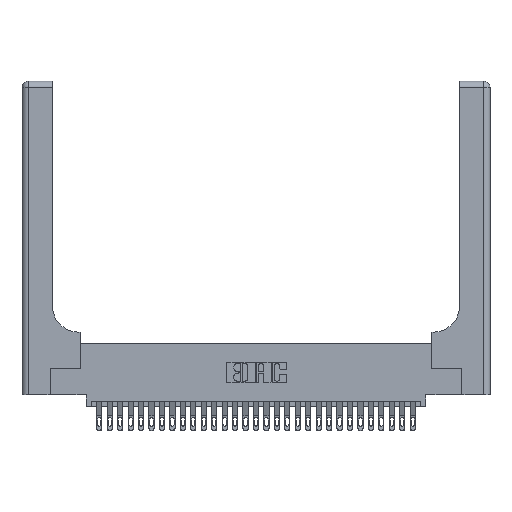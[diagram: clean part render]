
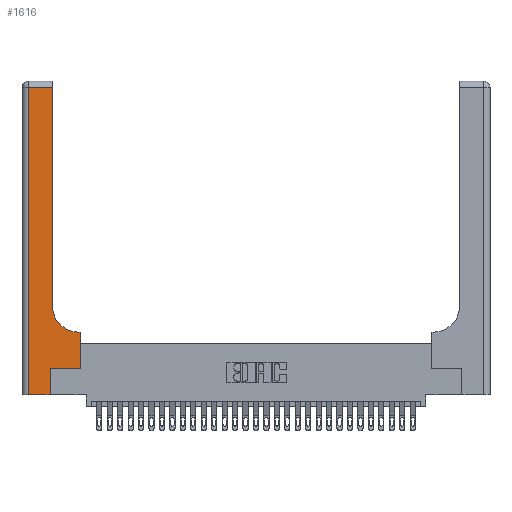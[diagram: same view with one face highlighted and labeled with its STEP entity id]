
A CAD part, top view. The second image highlights one B-rep face of the part: STEP entity #1616.
In plain terms, the highlighted planar face has unit normal (0, 0, 1).
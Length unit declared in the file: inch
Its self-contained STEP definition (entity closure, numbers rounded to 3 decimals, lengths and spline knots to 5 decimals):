
#83 = VERTEX_POINT ( 'NONE', #4562 ) ;
#163 = CARTESIAN_POINT ( 'NONE',  ( 0., 2.94, 0.37 ) ) ;
#484 = DIRECTION ( 'NONE',  ( 0., 1., 0. ) ) ;
#502 = EDGE_CURVE ( 'NONE', #7947, #1816, #18772, .T. ) ;
#933 = VERTEX_POINT ( 'NONE', #20102 ) ;
#1616 = ADVANCED_FACE ( 'NONE', ( #16328 ), #7703, .F. ) ;
#1675 = DIRECTION ( 'NONE',  ( 1., 0., 0. ) ) ;
#1691 = CARTESIAN_POINT ( 'NONE',  ( 0.06, 3., 0.37 ) ) ;
#1816 = VERTEX_POINT ( 'NONE', #5669 ) ;
#2248 = ORIENTED_EDGE ( 'NONE', *, *, #26044, .T. ) ;
#2828 = EDGE_CURVE ( 'NONE', #26801, #7947, #7491, .T. ) ;
#3891 = VECTOR ( 'NONE', #13024, 39.37008 ) ;
#3899 = DIRECTION ( 'NONE',  ( 1., 0., 0. ) ) ;
#4047 = CARTESIAN_POINT ( 'NONE',  ( 0.269, 0., 0.37 ) ) ;
#4562 = CARTESIAN_POINT ( 'NONE',  ( 0.269, 0.25, 0.37 ) ) ;
#4791 = LINE ( 'NONE', #13809, #12386 ) ;
#4873 = CARTESIAN_POINT ( 'NONE',  ( 0.2915, 0.6, 0.37 ) ) ;
#4893 = AXIS2_PLACEMENT_3D ( 'NONE', #7913, #24890, #27319 ) ;
#4929 = ORIENTED_EDGE ( 'NONE', *, *, #8617, .T. ) ;
#5489 = AXIS2_PLACEMENT_3D ( 'NONE', #18535, #18327, #3899 ) ;
#5669 = CARTESIAN_POINT ( 'NONE',  ( 0.2915, 0.85, 0.37 ) ) ;
#6966 = VECTOR ( 'NONE', #21246, 39.37008 ) ;
#7172 = ORIENTED_EDGE ( 'NONE', *, *, #28319, .T. ) ;
#7491 = LINE ( 'NONE', #4873, #17726 ) ;
#7548 = VECTOR ( 'NONE', #10978, 39.37008 ) ;
#7703 = PLANE ( 'NONE',  #4893 ) ;
#7913 = CARTESIAN_POINT ( 'NONE',  ( 0., 3., 0.37 ) ) ;
#7947 = VERTEX_POINT ( 'NONE', #29846 ) ;
#8249 = CARTESIAN_POINT ( 'NONE',  ( 0., 0., 0.37 ) ) ;
#8617 = EDGE_CURVE ( 'NONE', #10049, #933, #21495, .T. ) ;
#9253 = ORIENTED_EDGE ( 'NONE', *, *, #10147, .T. ) ;
#9971 = CARTESIAN_POINT ( 'NONE',  ( 0.5585, 0.25, 0.37 ) ) ;
#10049 = VERTEX_POINT ( 'NONE', #26014 ) ;
#10147 = EDGE_CURVE ( 'NONE', #933, #15327, #12277, .T. ) ;
#10602 = LINE ( 'NONE', #13424, #7548 ) ;
#10978 = DIRECTION ( 'NONE',  ( 0., 1., 0. ) ) ;
#11317 = ORIENTED_EDGE ( 'NONE', *, *, #12774, .T. ) ;
#11556 = EDGE_CURVE ( 'NONE', #15327, #11766, #29725, .T. ) ;
#11766 = VERTEX_POINT ( 'NONE', #21066 ) ;
#12277 = LINE ( 'NONE', #1691, #16464 ) ;
#12386 = VECTOR ( 'NONE', #1675, 39.37008 ) ;
#12774 = EDGE_CURVE ( 'NONE', #25693, #26801, #28113, .T. ) ;
#13024 = DIRECTION ( 'NONE',  ( 1., 0., 0. ) ) ;
#13424 = CARTESIAN_POINT ( 'NONE',  ( 0.2915, 3., 0.37 ) ) ;
#13809 = CARTESIAN_POINT ( 'NONE',  ( 0.269, 0.25, 0.37 ) ) ;
#14570 = ORIENTED_EDGE ( 'NONE', *, *, #502, .T. ) ;
#14626 = EDGE_LOOP ( 'NONE', ( #25758, #4929, #9253, #25588, #2248, #7172, #11317, #18709, #14570 ) ) ;
#15271 = EDGE_CURVE ( 'NONE', #1816, #10049, #10602, .T. ) ;
#15327 = VERTEX_POINT ( 'NONE', #17867 ) ;
#16328 = FACE_OUTER_BOUND ( 'NONE', #14626, .T. ) ;
#16464 = VECTOR ( 'NONE', #26918, 39.37008 ) ;
#17178 = DIRECTION ( 'NONE',  ( -1., 0., 0. ) ) ;
#17726 = VECTOR ( 'NONE', #26832, 39.37008 ) ;
#17867 = CARTESIAN_POINT ( 'NONE',  ( 0.06, 0., 0.37 ) ) ;
#18327 = DIRECTION ( 'NONE',  ( 0., 0., -1. ) ) ;
#18535 = CARTESIAN_POINT ( 'NONE',  ( 0.5415, 0.85, 0.37 ) ) ;
#18709 = ORIENTED_EDGE ( 'NONE', *, *, #2828, .T. ) ;
#18772 = CIRCLE ( 'NONE', #5489, 0.25 ) ;
#20102 = CARTESIAN_POINT ( 'NONE',  ( 0.06, 2.94, 0.37 ) ) ;
#21066 = CARTESIAN_POINT ( 'NONE',  ( 0.269, 0., 0.37 ) ) ;
#21246 = DIRECTION ( 'NONE',  ( 0., 1., 0. ) ) ;
#21495 = LINE ( 'NONE', #163, #26056 ) ;
#23568 = VECTOR ( 'NONE', #484, 39.37008 ) ;
#24815 = LINE ( 'NONE', #4047, #6966 ) ;
#24890 = DIRECTION ( 'NONE',  ( 0., 0., -1. ) ) ;
#25081 = CARTESIAN_POINT ( 'NONE',  ( 0.5585, 0.25, 0.37 ) ) ;
#25588 = ORIENTED_EDGE ( 'NONE', *, *, #11556, .T. ) ;
#25693 = VERTEX_POINT ( 'NONE', #25081 ) ;
#25758 = ORIENTED_EDGE ( 'NONE', *, *, #15271, .T. ) ;
#26014 = CARTESIAN_POINT ( 'NONE',  ( 0.2915, 2.94, 0.37 ) ) ;
#26044 = EDGE_CURVE ( 'NONE', #11766, #83, #24815, .T. ) ;
#26056 = VECTOR ( 'NONE', #17178, 39.37008 ) ;
#26801 = VERTEX_POINT ( 'NONE', #31163 ) ;
#26832 = DIRECTION ( 'NONE',  ( -1., 0., 0. ) ) ;
#26918 = DIRECTION ( 'NONE',  ( 0., -1., 0. ) ) ;
#27319 = DIRECTION ( 'NONE',  ( -1., 0., 0. ) ) ;
#28113 = LINE ( 'NONE', #9971, #23568 ) ;
#28319 = EDGE_CURVE ( 'NONE', #83, #25693, #4791, .T. ) ;
#29725 = LINE ( 'NONE', #8249, #3891 ) ;
#29846 = CARTESIAN_POINT ( 'NONE',  ( 0.5415, 0.6, 0.37 ) ) ;
#31163 = CARTESIAN_POINT ( 'NONE',  ( 0.5585, 0.6, 0.37 ) ) ;
